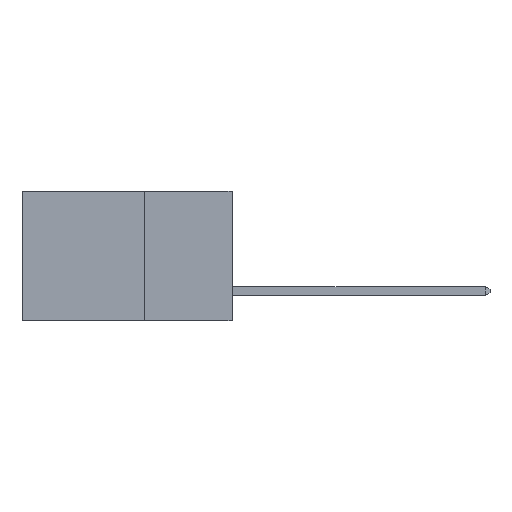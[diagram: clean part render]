
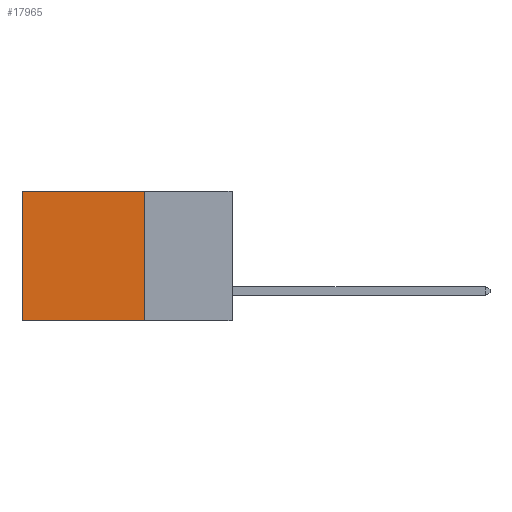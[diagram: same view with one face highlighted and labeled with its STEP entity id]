
A CAD part, left-side view. The second image highlights one B-rep face of the part: STEP entity #17965.
In plain terms, the highlighted planar face has unit normal (-1, 0, 0).
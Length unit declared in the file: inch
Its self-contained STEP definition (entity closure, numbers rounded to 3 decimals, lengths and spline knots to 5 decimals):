
#1701 = EDGE_CURVE ( 'NONE', #11952, #6003, #23747, .T. ) ;
#1794 = FACE_OUTER_BOUND ( 'NONE', #10634, .T. ) ;
#2036 = VECTOR ( 'NONE', #22426, 39.37008 ) ;
#2520 = CARTESIAN_POINT ( 'NONE',  ( 0.2875, 0.6, 0. ) ) ;
#5141 = CARTESIAN_POINT ( 'NONE',  ( 0.2875, 0.25, -0.37 ) ) ;
#6003 = VERTEX_POINT ( 'NONE', #17194 ) ;
#6626 = PLANE ( 'NONE',  #12390 ) ;
#6741 = CARTESIAN_POINT ( 'NONE',  ( 0.2875, 0.25, 0. ) ) ;
#7344 = ORIENTED_EDGE ( 'NONE', *, *, #1701, .F. ) ;
#7801 = LINE ( 'NONE', #24152, #12338 ) ;
#7831 = LINE ( 'NONE', #14695, #2036 ) ;
#8206 = VECTOR ( 'NONE', #20701, 39.37008 ) ;
#8489 = CARTESIAN_POINT ( 'NONE',  ( 0.2875, 0.25, 0. ) ) ;
#8570 = DIRECTION ( 'NONE',  ( 1., 0., 0. ) ) ;
#8737 = EDGE_CURVE ( 'NONE', #11541, #6003, #9313, .T. ) ;
#9313 = LINE ( 'NONE', #15489, #24837 ) ;
#10634 = EDGE_LOOP ( 'NONE', ( #15102, #7344, #12246, #16409 ) ) ;
#11541 = VERTEX_POINT ( 'NONE', #2520 ) ;
#11952 = VERTEX_POINT ( 'NONE', #19257 ) ;
#12246 = ORIENTED_EDGE ( 'NONE', *, *, #19018, .F. ) ;
#12338 = VECTOR ( 'NONE', #18368, 39.37008 ) ;
#12390 = AXIS2_PLACEMENT_3D ( 'NONE', #8489, #8570, #22194 ) ;
#13608 = EDGE_CURVE ( 'NONE', #19605, #11541, #7801, .T. ) ;
#14695 = CARTESIAN_POINT ( 'NONE',  ( 0.2875, 0.25, 0. ) ) ;
#15102 = ORIENTED_EDGE ( 'NONE', *, *, #8737, .T. ) ;
#15489 = CARTESIAN_POINT ( 'NONE',  ( 0.2875, 0.6, 0. ) ) ;
#16409 = ORIENTED_EDGE ( 'NONE', *, *, #13608, .T. ) ;
#17194 = CARTESIAN_POINT ( 'NONE',  ( 0.2875, 0.6, -0.37 ) ) ;
#17435 = DIRECTION ( 'NONE',  ( 0., 0., -1. ) ) ;
#17965 = ADVANCED_FACE ( 'NONE', ( #1794 ), #6626, .F. ) ;
#18368 = DIRECTION ( 'NONE',  ( 0., 1., 0. ) ) ;
#19018 = EDGE_CURVE ( 'NONE', #19605, #11952, #7831, .T. ) ;
#19257 = CARTESIAN_POINT ( 'NONE',  ( 0.2875, 0.25, -0.37 ) ) ;
#19605 = VERTEX_POINT ( 'NONE', #6741 ) ;
#20701 = DIRECTION ( 'NONE',  ( 0., 1., 0. ) ) ;
#22194 = DIRECTION ( 'NONE',  ( 0., 0., -1. ) ) ;
#22426 = DIRECTION ( 'NONE',  ( 0., 0., -1. ) ) ;
#23747 = LINE ( 'NONE', #5141, #8206 ) ;
#24152 = CARTESIAN_POINT ( 'NONE',  ( 0.2875, 0.25, 0. ) ) ;
#24837 = VECTOR ( 'NONE', #17435, 39.37008 ) ;
